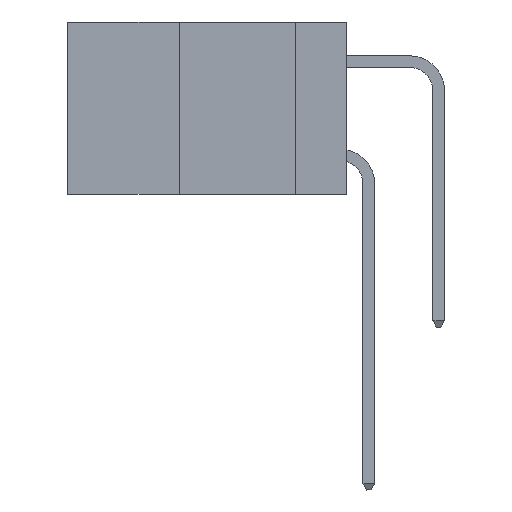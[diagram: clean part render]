
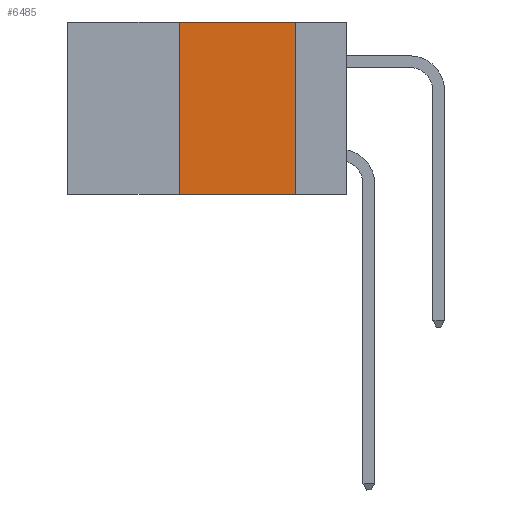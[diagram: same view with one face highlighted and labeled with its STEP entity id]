
A CAD part, left-side view. The second image highlights one B-rep face of the part: STEP entity #6485.
In plain terms, the highlighted planar face has unit normal (-1, 0, 0).
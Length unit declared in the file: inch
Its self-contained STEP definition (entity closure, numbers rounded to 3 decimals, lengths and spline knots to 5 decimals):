
#121 = EDGE_CURVE ( 'NONE', #7303, #2301, #6967, .T. ) ;
#264 = CARTESIAN_POINT ( 'NONE',  ( 0., 0.36, 0. ) ) ;
#343 = DIRECTION ( 'NONE',  ( 0., 0., -1. ) ) ;
#412 = CARTESIAN_POINT ( 'NONE',  ( 0., 0.6, 0. ) ) ;
#471 = DIRECTION ( 'NONE',  ( 0., -1., 0. ) ) ;
#1116 = DIRECTION ( 'NONE',  ( 1., 0., 0. ) ) ;
#1926 = LINE ( 'NONE', #12355, #13128 ) ;
#2301 = VERTEX_POINT ( 'NONE', #5157 ) ;
#3124 = VERTEX_POINT ( 'NONE', #13299 ) ;
#3269 = VECTOR ( 'NONE', #343, 39.37008 ) ;
#3794 = FACE_OUTER_BOUND ( 'NONE', #12288, .T. ) ;
#3843 = EDGE_CURVE ( 'NONE', #13354, #3124, #1926, .T. ) ;
#4588 = EDGE_CURVE ( 'NONE', #13354, #7303, #12346, .T. ) ;
#5157 = CARTESIAN_POINT ( 'NONE',  ( 0., 0.11, 0. ) ) ;
#5618 = CARTESIAN_POINT ( 'NONE',  ( 0., 0.6, 0. ) ) ;
#6165 = LINE ( 'NONE', #13216, #3269 ) ;
#6485 = ADVANCED_FACE ( 'NONE', ( #3794 ), #6672, .F. ) ;
#6552 = ORIENTED_EDGE ( 'NONE', *, *, #6738, .F. ) ;
#6672 = PLANE ( 'NONE',  #10710 ) ;
#6738 = EDGE_CURVE ( 'NONE', #2301, #3124, #6165, .T. ) ;
#6967 = LINE ( 'NONE', #412, #9424 ) ;
#7203 = VECTOR ( 'NONE', #7919, 39.37008 ) ;
#7303 = VERTEX_POINT ( 'NONE', #264 ) ;
#7919 = DIRECTION ( 'NONE',  ( 0., 0., 1. ) ) ;
#8788 = DIRECTION ( 'NONE',  ( 0., 0., -1. ) ) ;
#9424 = VECTOR ( 'NONE', #471, 39.37008 ) ;
#10098 = DIRECTION ( 'NONE',  ( 0., -1., 0. ) ) ;
#10180 = ORIENTED_EDGE ( 'NONE', *, *, #4588, .F. ) ;
#10710 = AXIS2_PLACEMENT_3D ( 'NONE', #5618, #1116, #8788 ) ;
#11690 = CARTESIAN_POINT ( 'NONE',  ( 0., 0.36, 0. ) ) ;
#11760 = ORIENTED_EDGE ( 'NONE', *, *, #121, .F. ) ;
#12288 = EDGE_LOOP ( 'NONE', ( #6552, #11760, #10180, #12542 ) ) ;
#12346 = LINE ( 'NONE', #11690, #7203 ) ;
#12355 = CARTESIAN_POINT ( 'NONE',  ( 0., 0.6, -0.37 ) ) ;
#12542 = ORIENTED_EDGE ( 'NONE', *, *, #3843, .T. ) ;
#13128 = VECTOR ( 'NONE', #10098, 39.37008 ) ;
#13216 = CARTESIAN_POINT ( 'NONE',  ( 0., 0.11, 0. ) ) ;
#13299 = CARTESIAN_POINT ( 'NONE',  ( 0., 0.11, -0.37 ) ) ;
#13354 = VERTEX_POINT ( 'NONE', #13524 ) ;
#13524 = CARTESIAN_POINT ( 'NONE',  ( 0., 0.36, -0.37 ) ) ;
